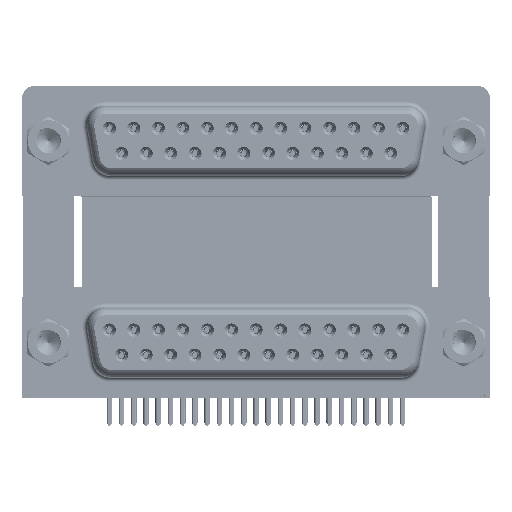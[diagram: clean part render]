
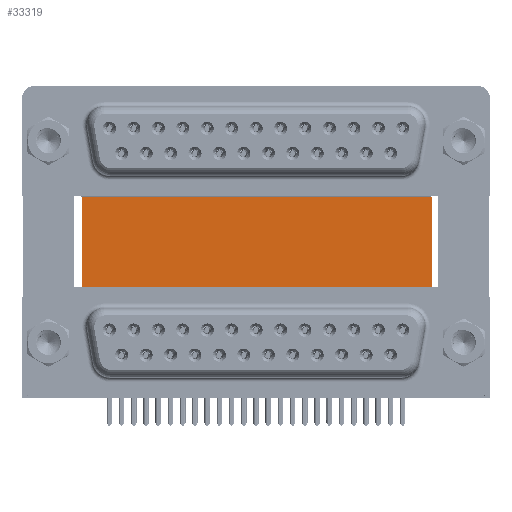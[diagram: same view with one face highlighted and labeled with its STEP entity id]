
A CAD part, top view. The second image highlights one B-rep face of the part: STEP entity #33319.
In plain terms, the highlighted planar face has unit normal (0, 0, 1).
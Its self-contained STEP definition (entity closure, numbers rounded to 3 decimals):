
#7314 = FACE_OUTER_BOUND ( 'NONE', #64603, .T. ) ;
#7661 = DIRECTION ( 'NONE',  ( -1., 0., 0. ) ) ;
#8223 = ORIENTED_EDGE ( 'NONE', *, *, #45305, .F. ) ;
#11435 = DIRECTION ( 'NONE',  ( 0., 0., -1. ) ) ;
#12631 = DIRECTION ( 'NONE',  ( 0., -1., 0. ) ) ;
#18621 = CARTESIAN_POINT ( 'NONE',  ( 43.43, -3.735, -12. ) ) ;
#18796 = VERTEX_POINT ( 'NONE', #33527 ) ;
#19639 = EDGE_CURVE ( 'NONE', #56905, #28781, #22760, .T. ) ;
#22760 = LINE ( 'NONE', #32684, #63581 ) ;
#24904 = ORIENTED_EDGE ( 'NONE', *, *, #19639, .T. ) ;
#24934 = EDGE_CURVE ( 'NONE', #18796, #56905, #46137, .T. ) ;
#26150 = EDGE_CURVE ( 'NONE', #18796, #31554, #50954, .T. ) ;
#28563 = PLANE ( 'NONE',  #41484 ) ;
#28781 = VERTEX_POINT ( 'NONE', #18621 ) ;
#31554 = VERTEX_POINT ( 'NONE', #35390 ) ;
#32513 = LINE ( 'NONE', #58197, #51962 ) ;
#32684 = CARTESIAN_POINT ( 'NONE',  ( 3.79, -3.735, -12. ) ) ;
#33319 = ADVANCED_FACE ( 'NONE', ( #7314 ), #28563, .F. ) ;
#33527 = CARTESIAN_POINT ( 'NONE',  ( 3.79, 16.585, -12. ) ) ;
#34331 = VECTOR ( 'NONE', #57083, 1000. ) ;
#35390 = CARTESIAN_POINT ( 'NONE',  ( 43.43, 16.585, -12. ) ) ;
#37880 = DIRECTION ( 'NONE',  ( 1., 0., 0. ) ) ;
#41484 = AXIS2_PLACEMENT_3D ( 'NONE', #64529, #11435, #7661 ) ;
#43968 = DIRECTION ( 'NONE',  ( 1., 0., 0. ) ) ;
#45305 = EDGE_CURVE ( 'NONE', #31554, #28781, #32513, .T. ) ;
#46137 = LINE ( 'NONE', #52272, #34331 ) ;
#47525 = VECTOR ( 'NONE', #37880, 1000. ) ;
#47836 = CARTESIAN_POINT ( 'NONE',  ( 3.79, 16.585, -12. ) ) ;
#48001 = ORIENTED_EDGE ( 'NONE', *, *, #26150, .F. ) ;
#50954 = LINE ( 'NONE', #47836, #47525 ) ;
#51962 = VECTOR ( 'NONE', #12631, 1000. ) ;
#52272 = CARTESIAN_POINT ( 'NONE',  ( 3.79, 16.585, -12. ) ) ;
#56905 = VERTEX_POINT ( 'NONE', #58253 ) ;
#57083 = DIRECTION ( 'NONE',  ( 0., -1., 0. ) ) ;
#58197 = CARTESIAN_POINT ( 'NONE',  ( 43.43, 16.585, -12. ) ) ;
#58253 = CARTESIAN_POINT ( 'NONE',  ( 3.79, -3.735, -12. ) ) ;
#63581 = VECTOR ( 'NONE', #43968, 1000. ) ;
#64529 = CARTESIAN_POINT ( 'NONE',  ( 3.79, 16.585, -12. ) ) ;
#64603 = EDGE_LOOP ( 'NONE', ( #24904, #8223, #48001, #65111 ) ) ;
#65111 = ORIENTED_EDGE ( 'NONE', *, *, #24934, .T. ) ;
